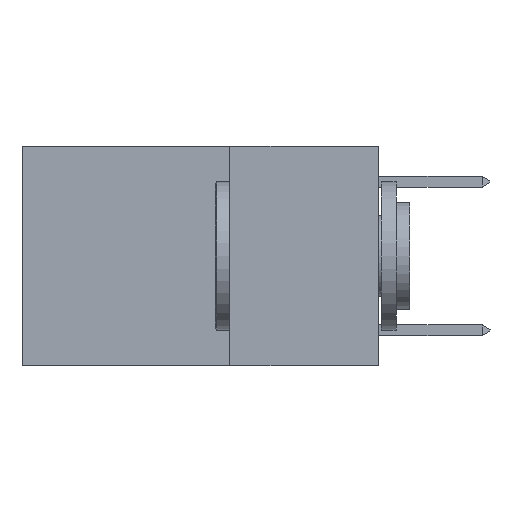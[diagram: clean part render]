
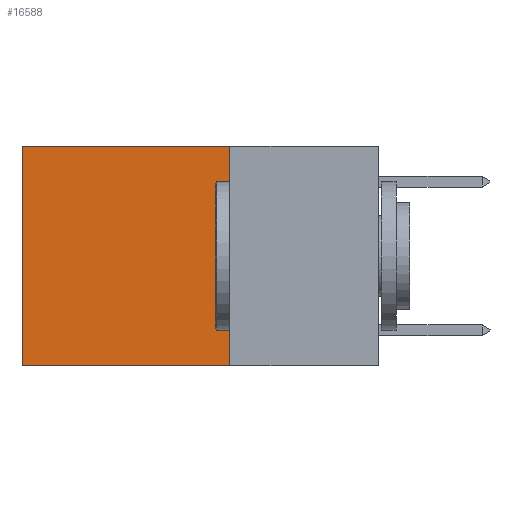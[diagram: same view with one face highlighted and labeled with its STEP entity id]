
A CAD part, left-side view. The second image highlights one B-rep face of the part: STEP entity #16588.
In plain terms, the highlighted planar face has unit normal (-1, 0, 0).
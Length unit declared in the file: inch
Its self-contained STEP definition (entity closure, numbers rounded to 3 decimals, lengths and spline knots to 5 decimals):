
#2671 = PLANE ( 'NONE',  #9918 ) ;
#3360 = FACE_OUTER_BOUND ( 'NONE', #18990, .T. ) ;
#3595 = ORIENTED_EDGE ( 'NONE', *, *, #21400, .F. ) ;
#3906 = VERTEX_POINT ( 'NONE', #11556 ) ;
#4288 = CARTESIAN_POINT ( 'NONE',  ( 0.2625, 0.6, -0.37 ) ) ;
#4586 = DIRECTION ( 'NONE',  ( 0., 0., -1. ) ) ;
#7104 = CARTESIAN_POINT ( 'NONE',  ( 0.2625, 0.25, -0.37 ) ) ;
#7884 = CARTESIAN_POINT ( 'NONE',  ( 0.2625, 0.6, 0. ) ) ;
#8428 = CARTESIAN_POINT ( 'NONE',  ( 0.2625, 0.25, 0. ) ) ;
#9918 = AXIS2_PLACEMENT_3D ( 'NONE', #20844, #15541, #4586 ) ;
#10266 = DIRECTION ( 'NONE',  ( 0., 0., -1. ) ) ;
#11556 = CARTESIAN_POINT ( 'NONE',  ( 0.2625, 0.25, 0. ) ) ;
#12336 = VECTOR ( 'NONE', #12621, 39.37008 ) ;
#12483 = LINE ( 'NONE', #23514, #12917 ) ;
#12551 = LINE ( 'NONE', #7104, #12336 ) ;
#12621 = DIRECTION ( 'NONE',  ( 0., 1., 0. ) ) ;
#12917 = VECTOR ( 'NONE', #16678, 39.37008 ) ;
#14497 = VECTOR ( 'NONE', #10266, 39.37008 ) ;
#14534 = EDGE_CURVE ( 'NONE', #17325, #18582, #15808, .T. ) ;
#14707 = LINE ( 'NONE', #8428, #14497 ) ;
#14943 = EDGE_CURVE ( 'NONE', #3906, #17325, #12483, .T. ) ;
#15541 = DIRECTION ( 'NONE',  ( 1., 0., 0. ) ) ;
#15808 = LINE ( 'NONE', #7884, #15872 ) ;
#15872 = VECTOR ( 'NONE', #20539, 39.37008 ) ;
#16588 = ADVANCED_FACE ( 'NONE', ( #3360 ), #2671, .F. ) ;
#16678 = DIRECTION ( 'NONE',  ( 0., 1., 0. ) ) ;
#17325 = VERTEX_POINT ( 'NONE', #20968 ) ;
#18582 = VERTEX_POINT ( 'NONE', #4288 ) ;
#18990 = EDGE_LOOP ( 'NONE', ( #20613, #3595, #19650, #20597 ) ) ;
#19650 = ORIENTED_EDGE ( 'NONE', *, *, #22466, .F. ) ;
#20539 = DIRECTION ( 'NONE',  ( 0., 0., -1. ) ) ;
#20597 = ORIENTED_EDGE ( 'NONE', *, *, #14943, .T. ) ;
#20613 = ORIENTED_EDGE ( 'NONE', *, *, #14534, .T. ) ;
#20844 = CARTESIAN_POINT ( 'NONE',  ( 0.2625, 0.25, 0. ) ) ;
#20968 = CARTESIAN_POINT ( 'NONE',  ( 0.2625, 0.6, 0. ) ) ;
#21400 = EDGE_CURVE ( 'NONE', #21421, #18582, #12551, .T. ) ;
#21421 = VERTEX_POINT ( 'NONE', #23198 ) ;
#22466 = EDGE_CURVE ( 'NONE', #3906, #21421, #14707, .T. ) ;
#23198 = CARTESIAN_POINT ( 'NONE',  ( 0.2625, 0.25, -0.37 ) ) ;
#23514 = CARTESIAN_POINT ( 'NONE',  ( 0.2625, 0.25, 0. ) ) ;
